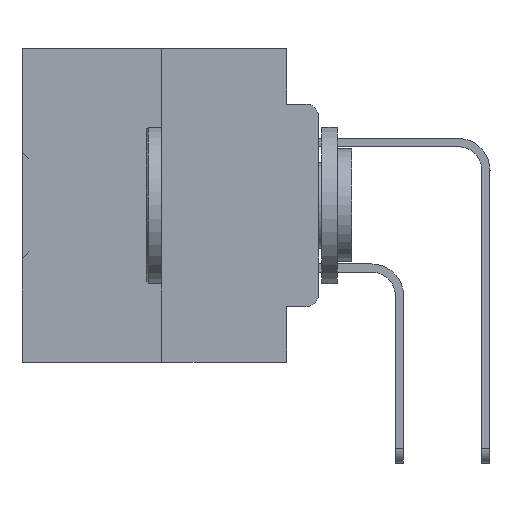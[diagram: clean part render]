
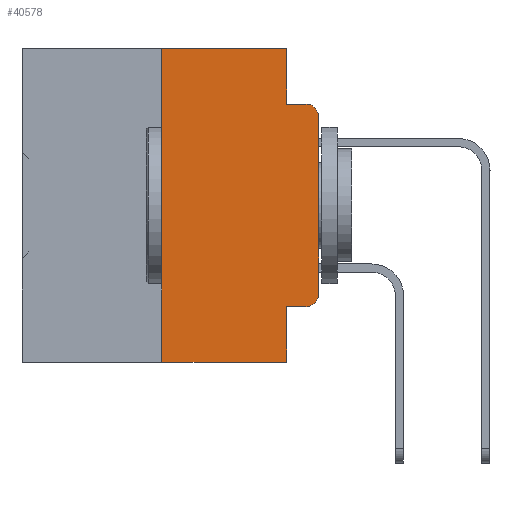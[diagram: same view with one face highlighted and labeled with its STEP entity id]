
A CAD part, left-side view. The second image highlights one B-rep face of the part: STEP entity #40578.
In plain terms, the highlighted planar face has unit normal (-1, 0, 0).
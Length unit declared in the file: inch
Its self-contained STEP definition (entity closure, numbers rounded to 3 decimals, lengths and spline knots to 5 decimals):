
#91 = VECTOR ( 'NONE', #27463, 39.37008 ) ;
#198 = CARTESIAN_POINT ( 'NONE',  ( 0., 0.051, -0.0885 ) ) ;
#247 = VECTOR ( 'NONE', #17295, 39.37008 ) ;
#357 = ORIENTED_EDGE ( 'NONE', *, *, #26662, .F. ) ;
#511 = CARTESIAN_POINT ( 'NONE',  ( 0., 0.051, -0.0885 ) ) ;
#1411 = EDGE_CURVE ( 'NONE', #24669, #6237, #22078, .T. ) ;
#1732 = LINE ( 'NONE', #8540, #91 ) ;
#1841 = ORIENTED_EDGE ( 'NONE', *, *, #28355, .F. ) ;
#2394 = DIRECTION ( 'NONE',  ( 0., 0., 1. ) ) ;
#2510 = VECTOR ( 'NONE', #14798, 39.37008 ) ;
#3803 = DIRECTION ( 'NONE',  ( 0., 0., -1. ) ) ;
#3867 = LINE ( 'NONE', #4060, #33800 ) ;
#4060 = CARTESIAN_POINT ( 'NONE',  ( 0., 0.051, -0.4115 ) ) ;
#4934 = VERTEX_POINT ( 'NONE', #27990 ) ;
#6237 = VERTEX_POINT ( 'NONE', #21633 ) ;
#6495 = DIRECTION ( 'NONE',  ( -1., 0., 0. ) ) ;
#6796 = ORIENTED_EDGE ( 'NONE', *, *, #25929, .F. ) ;
#7251 = DIRECTION ( 'NONE',  ( 1., 0., 0. ) ) ;
#8386 = CARTESIAN_POINT ( 'NONE',  ( 0., 0., -0.3915 ) ) ;
#8540 = CARTESIAN_POINT ( 'NONE',  ( 0., 0.051, 0. ) ) ;
#9893 = ORIENTED_EDGE ( 'NONE', *, *, #11023, .F. ) ;
#9969 = CARTESIAN_POINT ( 'NONE',  ( 0., 0.051, 0. ) ) ;
#10595 = ORIENTED_EDGE ( 'NONE', *, *, #32865, .F. ) ;
#11023 = EDGE_CURVE ( 'NONE', #4934, #17142, #25290, .T. ) ;
#11099 = VERTEX_POINT ( 'NONE', #38026 ) ;
#12144 = CARTESIAN_POINT ( 'NONE',  ( 0., 0.051, 0. ) ) ;
#12257 = LINE ( 'NONE', #9969, #18204 ) ;
#13071 = CARTESIAN_POINT ( 'NONE',  ( 0., 0.02, -0.3915 ) ) ;
#13285 = LINE ( 'NONE', #511, #25933 ) ;
#14798 = DIRECTION ( 'NONE',  ( 0., -1., 0. ) ) ;
#15326 = CARTESIAN_POINT ( 'NONE',  ( 0., 0.02, -0.1085 ) ) ;
#15452 = VERTEX_POINT ( 'NONE', #8386 ) ;
#15567 = LINE ( 'NONE', #18865, #17991 ) ;
#16288 = AXIS2_PLACEMENT_3D ( 'NONE', #15326, #40003, #25185 ) ;
#16620 = DIRECTION ( 'NONE',  ( 0., -1., 0. ) ) ;
#17142 = VERTEX_POINT ( 'NONE', #12144 ) ;
#17223 = CARTESIAN_POINT ( 'NONE',  ( 0., 0.02, -0.4115 ) ) ;
#17295 = DIRECTION ( 'NONE',  ( 0., 0., 1. ) ) ;
#17330 = CARTESIAN_POINT ( 'NONE',  ( 0., 0.473, 0. ) ) ;
#17991 = VECTOR ( 'NONE', #2394, 39.37008 ) ;
#18204 = VECTOR ( 'NONE', #28474, 39.37008 ) ;
#18865 = CARTESIAN_POINT ( 'NONE',  ( 0., 0., 0. ) ) ;
#19377 = DIRECTION ( 'NONE',  ( 0., -1., 0. ) ) ;
#19463 = AXIS2_PLACEMENT_3D ( 'NONE', #13071, #6495, #3803 ) ;
#19812 = DIRECTION ( 'NONE',  ( 0., 0., -1. ) ) ;
#21633 = CARTESIAN_POINT ( 'NONE',  ( 0., 0.051, -0.5 ) ) ;
#21662 = VECTOR ( 'NONE', #19377, 39.37008 ) ;
#22078 = LINE ( 'NONE', #28036, #21662 ) ;
#22229 = CIRCLE ( 'NONE', #16288, 0.02 ) ;
#22376 = EDGE_CURVE ( 'NONE', #23598, #38033, #22229, .T. ) ;
#22612 = CARTESIAN_POINT ( 'NONE',  ( 0., 0.473, 0. ) ) ;
#23598 = VERTEX_POINT ( 'NONE', #24405 ) ;
#23681 = LINE ( 'NONE', #29820, #247 ) ;
#23715 = PLANE ( 'NONE',  #34633 ) ;
#24405 = CARTESIAN_POINT ( 'NONE',  ( 0., 0., -0.1085 ) ) ;
#24669 = VERTEX_POINT ( 'NONE', #32826 ) ;
#24742 = VERTEX_POINT ( 'NONE', #17223 ) ;
#25185 = DIRECTION ( 'NONE',  ( 0., 0., -1. ) ) ;
#25290 = LINE ( 'NONE', #22612, #2510 ) ;
#25648 = ORIENTED_EDGE ( 'NONE', *, *, #37457, .T. ) ;
#25929 = EDGE_CURVE ( 'NONE', #24669, #4934, #23681, .T. ) ;
#25933 = VECTOR ( 'NONE', #35292, 39.37008 ) ;
#26320 = EDGE_CURVE ( 'NONE', #11099, #24742, #3867, .T. ) ;
#26662 = EDGE_CURVE ( 'NONE', #36623, #38033, #13285, .T. ) ;
#27463 = DIRECTION ( 'NONE',  ( 0., 0., -1. ) ) ;
#27990 = CARTESIAN_POINT ( 'NONE',  ( 0., 0.25, 0. ) ) ;
#28036 = CARTESIAN_POINT ( 'NONE',  ( 0., 0.473, -0.5 ) ) ;
#28355 = EDGE_CURVE ( 'NONE', #17142, #36623, #12257, .T. ) ;
#28474 = DIRECTION ( 'NONE',  ( 0., 0., -1. ) ) ;
#28999 = CARTESIAN_POINT ( 'NONE',  ( 0., 0.02, -0.0885 ) ) ;
#29037 = ORIENTED_EDGE ( 'NONE', *, *, #26320, .T. ) ;
#29820 = CARTESIAN_POINT ( 'NONE',  ( 0., 0.25, 0. ) ) ;
#31235 = ORIENTED_EDGE ( 'NONE', *, *, #1411, .T. ) ;
#32826 = CARTESIAN_POINT ( 'NONE',  ( 0., 0.25, -0.5 ) ) ;
#32865 = EDGE_CURVE ( 'NONE', #11099, #6237, #1732, .T. ) ;
#32950 = FACE_OUTER_BOUND ( 'NONE', #35060, .T. ) ;
#33259 = CIRCLE ( 'NONE', #19463, 0.02 ) ;
#33800 = VECTOR ( 'NONE', #16620, 39.37008 ) ;
#34633 = AXIS2_PLACEMENT_3D ( 'NONE', #17330, #7251, #19812 ) ;
#35007 = ORIENTED_EDGE ( 'NONE', *, *, #22376, .T. ) ;
#35060 = EDGE_LOOP ( 'NONE', ( #25648, #35007, #357, #1841, #9893, #6796, #31235, #10595, #29037, #36316 ) ) ;
#35292 = DIRECTION ( 'NONE',  ( 0., -1., 0. ) ) ;
#36316 = ORIENTED_EDGE ( 'NONE', *, *, #39902, .T. ) ;
#36623 = VERTEX_POINT ( 'NONE', #198 ) ;
#37457 = EDGE_CURVE ( 'NONE', #15452, #23598, #15567, .T. ) ;
#38026 = CARTESIAN_POINT ( 'NONE',  ( 0., 0.051, -0.4115 ) ) ;
#38033 = VERTEX_POINT ( 'NONE', #28999 ) ;
#39902 = EDGE_CURVE ( 'NONE', #24742, #15452, #33259, .T. ) ;
#40003 = DIRECTION ( 'NONE',  ( -1., 0., 0. ) ) ;
#40578 = ADVANCED_FACE ( 'NONE', ( #32950 ), #23715, .F. ) ;
